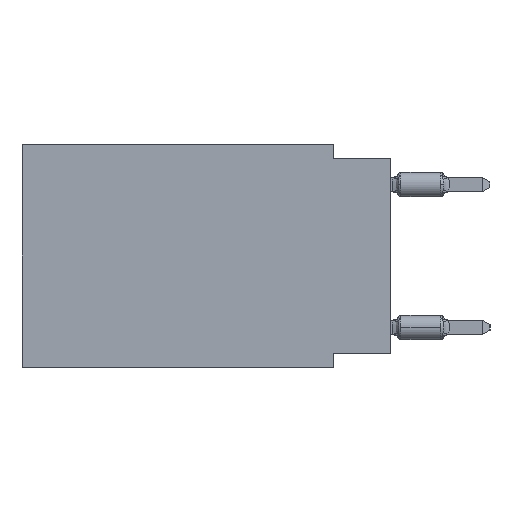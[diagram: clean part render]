
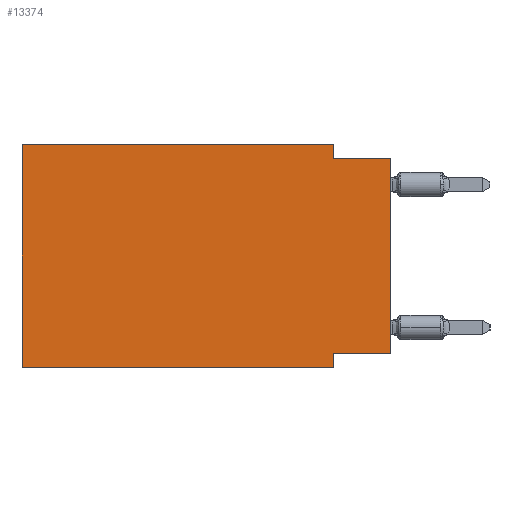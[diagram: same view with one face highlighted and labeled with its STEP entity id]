
A CAD part, left-side view. The second image highlights one B-rep face of the part: STEP entity #13374.
In plain terms, the highlighted planar face has unit normal (-1, 0, 0).
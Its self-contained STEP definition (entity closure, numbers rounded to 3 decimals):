
#859 = VERTEX_POINT ( 'NONE', #39257 ) ;
#921 = CARTESIAN_POINT ( 'NONE',  ( 0., 16.383, 0. ) ) ;
#1140 = FACE_OUTER_BOUND ( 'NONE', #37798, .T. ) ;
#1429 = CARTESIAN_POINT ( 'NONE',  ( 0., 2.54, -9.906 ) ) ;
#1755 = VERTEX_POINT ( 'NONE', #4146 ) ;
#2423 = CARTESIAN_POINT ( 'NONE',  ( 0., 2.54, 0. ) ) ;
#2518 = DIRECTION ( 'NONE',  ( 0., -1., 0. ) ) ;
#3176 = EDGE_CURVE ( 'NONE', #15364, #9092, #25790, .T. ) ;
#3438 = VERTEX_POINT ( 'NONE', #25119 ) ;
#3605 = ORIENTED_EDGE ( 'NONE', *, *, #37448, .T. ) ;
#4146 = CARTESIAN_POINT ( 'NONE',  ( 0., 2.54, -9.271 ) ) ;
#4340 = VERTEX_POINT ( 'NONE', #2423 ) ;
#4905 = LINE ( 'NONE', #8961, #38293 ) ;
#5297 = CARTESIAN_POINT ( 'NONE',  ( 0., 16.383, 0. ) ) ;
#6706 = VECTOR ( 'NONE', #28287, 1000. ) ;
#7178 = ORIENTED_EDGE ( 'NONE', *, *, #33299, .F. ) ;
#8961 = CARTESIAN_POINT ( 'NONE',  ( 0., 0., 0. ) ) ;
#9092 = VERTEX_POINT ( 'NONE', #37675 ) ;
#9165 = CARTESIAN_POINT ( 'NONE',  ( 0., 0., -0.635 ) ) ;
#9299 = ORIENTED_EDGE ( 'NONE', *, *, #16722, .F. ) ;
#10783 = ORIENTED_EDGE ( 'NONE', *, *, #3176, .T. ) ;
#11265 = EDGE_CURVE ( 'NONE', #3438, #1755, #31117, .T. ) ;
#12199 = ORIENTED_EDGE ( 'NONE', *, *, #21964, .F. ) ;
#12878 = VECTOR ( 'NONE', #19774, 1000. ) ;
#13374 = ADVANCED_FACE ( 'NONE', ( #1140 ), #20451, .F. ) ;
#14002 = DIRECTION ( 'NONE',  ( 0., 0., -1. ) ) ;
#14509 = LINE ( 'NONE', #1429, #16868 ) ;
#14598 = DIRECTION ( 'NONE',  ( 0., 1., 0. ) ) ;
#14810 = CARTESIAN_POINT ( 'NONE',  ( 0., 0., -9.271 ) ) ;
#15168 = EDGE_CURVE ( 'NONE', #4340, #36973, #15204, .T. ) ;
#15202 = LINE ( 'NONE', #9165, #30526 ) ;
#15204 = LINE ( 'NONE', #18205, #6706 ) ;
#15364 = VERTEX_POINT ( 'NONE', #26318 ) ;
#16722 = EDGE_CURVE ( 'NONE', #1755, #9092, #14509, .T. ) ;
#16868 = VECTOR ( 'NONE', #40679, 1000. ) ;
#18017 = CARTESIAN_POINT ( 'NONE',  ( 0., 2.54, -0.635 ) ) ;
#18205 = CARTESIAN_POINT ( 'NONE',  ( 0., 2.54, 0. ) ) ;
#19774 = DIRECTION ( 'NONE',  ( 0., -1., 0. ) ) ;
#20451 = PLANE ( 'NONE',  #40851 ) ;
#20784 = VECTOR ( 'NONE', #14598, 1000. ) ;
#21506 = CARTESIAN_POINT ( 'NONE',  ( 0., 16.383, 0. ) ) ;
#21675 = VECTOR ( 'NONE', #28664, 1000. ) ;
#21814 = LINE ( 'NONE', #5297, #22784 ) ;
#21964 = EDGE_CURVE ( 'NONE', #36973, #859, #15202, .T. ) ;
#22784 = VECTOR ( 'NONE', #35110, 1000. ) ;
#23917 = ORIENTED_EDGE ( 'NONE', *, *, #15168, .F. ) ;
#24805 = EDGE_CURVE ( 'NONE', #27338, #4340, #21814, .T. ) ;
#25119 = CARTESIAN_POINT ( 'NONE',  ( 0., 0., -9.271 ) ) ;
#25270 = DIRECTION ( 'NONE',  ( 0., 0., 1. ) ) ;
#25790 = LINE ( 'NONE', #35873, #12878 ) ;
#26318 = CARTESIAN_POINT ( 'NONE',  ( 0., 16.383, -9.906 ) ) ;
#26457 = ORIENTED_EDGE ( 'NONE', *, *, #11265, .F. ) ;
#27338 = VERTEX_POINT ( 'NONE', #21506 ) ;
#28063 = ORIENTED_EDGE ( 'NONE', *, *, #24805, .F. ) ;
#28287 = DIRECTION ( 'NONE',  ( 0., 0., -1. ) ) ;
#28664 = DIRECTION ( 'NONE',  ( 0., 0., 1. ) ) ;
#30526 = VECTOR ( 'NONE', #2518, 1000. ) ;
#31117 = LINE ( 'NONE', #14810, #20784 ) ;
#32298 = CARTESIAN_POINT ( 'NONE',  ( 0., 16.383, 0. ) ) ;
#33299 = EDGE_CURVE ( 'NONE', #15364, #27338, #41313, .T. ) ;
#35110 = DIRECTION ( 'NONE',  ( 0., -1., 0. ) ) ;
#35873 = CARTESIAN_POINT ( 'NONE',  ( 0., 16.383, -9.906 ) ) ;
#36958 = DIRECTION ( 'NONE',  ( 1., 0., 0. ) ) ;
#36973 = VERTEX_POINT ( 'NONE', #18017 ) ;
#37448 = EDGE_CURVE ( 'NONE', #3438, #859, #4905, .T. ) ;
#37675 = CARTESIAN_POINT ( 'NONE',  ( 0., 2.54, -9.906 ) ) ;
#37798 = EDGE_LOOP ( 'NONE', ( #3605, #12199, #23917, #28063, #7178, #10783, #9299, #26457 ) ) ;
#38293 = VECTOR ( 'NONE', #25270, 1000. ) ;
#39257 = CARTESIAN_POINT ( 'NONE',  ( 0., 0., -0.635 ) ) ;
#40679 = DIRECTION ( 'NONE',  ( 0., 0., -1. ) ) ;
#40851 = AXIS2_PLACEMENT_3D ( 'NONE', #921, #36958, #14002 ) ;
#41313 = LINE ( 'NONE', #32298, #21675 ) ;
